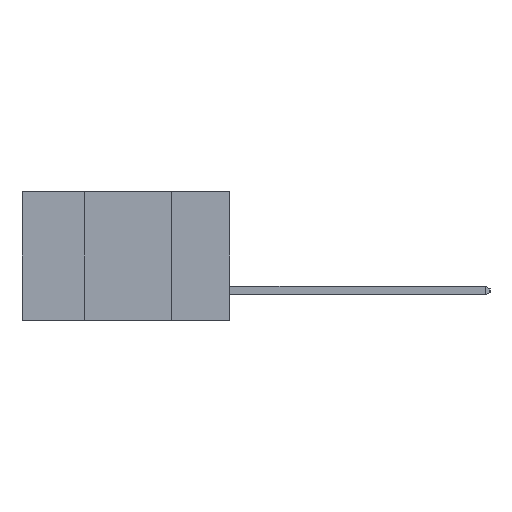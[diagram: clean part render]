
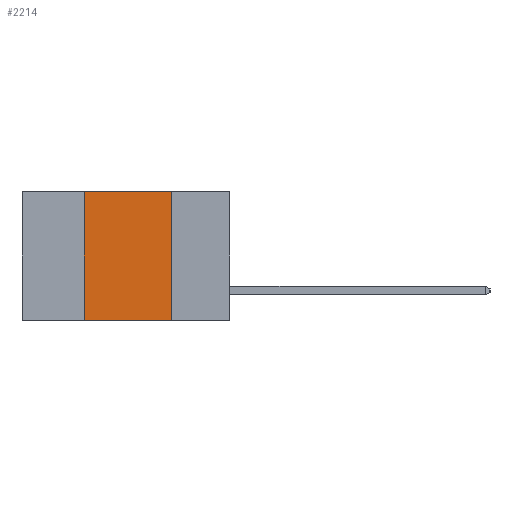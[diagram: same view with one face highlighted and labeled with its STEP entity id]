
A CAD part, left-side view. The second image highlights one B-rep face of the part: STEP entity #2214.
In plain terms, the highlighted planar face has unit normal (-1, 0, 0).
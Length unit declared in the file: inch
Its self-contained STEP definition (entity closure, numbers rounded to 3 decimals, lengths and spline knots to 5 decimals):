
#1322 = EDGE_CURVE ( 'NONE', #8704, #13502, #11006, .T. ) ;
#1732 = ORIENTED_EDGE ( 'NONE', *, *, #11008, .F. ) ;
#2214 = ADVANCED_FACE ( 'NONE', ( #13912 ), #14169, .F. ) ;
#2408 = VECTOR ( 'NONE', #15263, 39.37008 ) ;
#2636 = CARTESIAN_POINT ( 'NONE',  ( 0., 0.42, 0. ) ) ;
#3016 = LINE ( 'NONE', #12228, #19546 ) ;
#3414 = VECTOR ( 'NONE', #9875, 39.37008 ) ;
#4878 = ORIENTED_EDGE ( 'NONE', *, *, #18870, .F. ) ;
#5000 = ORIENTED_EDGE ( 'NONE', *, *, #19973, .F. ) ;
#5246 = CARTESIAN_POINT ( 'NONE',  ( 0., 0.42, -0.37 ) ) ;
#6361 = EDGE_LOOP ( 'NONE', ( #1732, #4878, #5000, #7405 ) ) ;
#6400 = VECTOR ( 'NONE', #9098, 39.37008 ) ;
#7405 = ORIENTED_EDGE ( 'NONE', *, *, #1322, .T. ) ;
#7756 = CARTESIAN_POINT ( 'NONE',  ( 0., 0.17, 0. ) ) ;
#8118 = CARTESIAN_POINT ( 'NONE',  ( 0., 0.6, -0.37 ) ) ;
#8704 = VERTEX_POINT ( 'NONE', #5246 ) ;
#8988 = AXIS2_PLACEMENT_3D ( 'NONE', #14258, #14044, #14004 ) ;
#9098 = DIRECTION ( 'NONE',  ( 0., -1., 0. ) ) ;
#9875 = DIRECTION ( 'NONE',  ( 0., 0., -1. ) ) ;
#10818 = VERTEX_POINT ( 'NONE', #7756 ) ;
#11006 = LINE ( 'NONE', #8118, #6400 ) ;
#11008 = EDGE_CURVE ( 'NONE', #10818, #13502, #17079, .T. ) ;
#11611 = CARTESIAN_POINT ( 'NONE',  ( 0., 0.17, -0.37 ) ) ;
#12228 = CARTESIAN_POINT ( 'NONE',  ( 0., 0.6, 0. ) ) ;
#13083 = CARTESIAN_POINT ( 'NONE',  ( 0., 0.17, -0.37 ) ) ;
#13502 = VERTEX_POINT ( 'NONE', #13083 ) ;
#13912 = FACE_OUTER_BOUND ( 'NONE', #6361, .T. ) ;
#14004 = DIRECTION ( 'NONE',  ( 0., 0., -1. ) ) ;
#14044 = DIRECTION ( 'NONE',  ( 1., 0., 0. ) ) ;
#14169 = PLANE ( 'NONE',  #8988 ) ;
#14258 = CARTESIAN_POINT ( 'NONE',  ( 0., 0.6, 0. ) ) ;
#15079 = LINE ( 'NONE', #20256, #2408 ) ;
#15263 = DIRECTION ( 'NONE',  ( 0., 0., 1. ) ) ;
#17079 = LINE ( 'NONE', #11611, #3414 ) ;
#18870 = EDGE_CURVE ( 'NONE', #21045, #10818, #3016, .T. ) ;
#19546 = VECTOR ( 'NONE', #20529, 39.37008 ) ;
#19973 = EDGE_CURVE ( 'NONE', #8704, #21045, #15079, .T. ) ;
#20256 = CARTESIAN_POINT ( 'NONE',  ( 0., 0.42, -0.37 ) ) ;
#20529 = DIRECTION ( 'NONE',  ( 0., -1., 0. ) ) ;
#21045 = VERTEX_POINT ( 'NONE', #2636 ) ;
